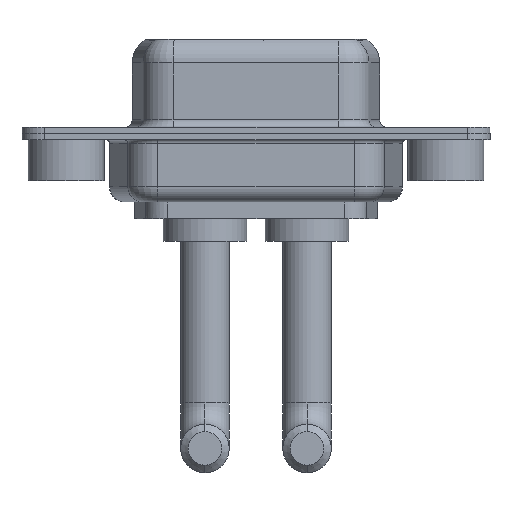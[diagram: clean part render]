
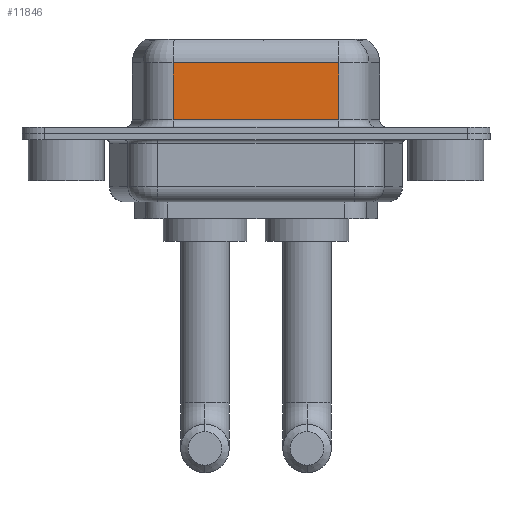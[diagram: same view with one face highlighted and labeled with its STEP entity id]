
A CAD part, front view. The second image highlights one B-rep face of the part: STEP entity #11846.
In plain terms, the highlighted planar face has unit normal (0, -1, 0).
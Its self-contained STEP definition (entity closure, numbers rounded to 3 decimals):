
#338 = CARTESIAN_POINT ( 'NONE',  ( 17.962, -3.95, 0.9 ) ) ;
#714 = VECTOR ( 'NONE', #4623, 1000. ) ;
#788 = VECTOR ( 'NONE', #2277, 1000. ) ;
#857 = CARTESIAN_POINT ( 'NONE',  ( 7.038, -3.95, 6.4 ) ) ;
#1573 = CARTESIAN_POINT ( 'NONE',  ( 17.962, -3.95, 4.65 ) ) ;
#1780 = DIRECTION ( 'NONE',  ( 0., 1., 0. ) ) ;
#1910 = DIRECTION ( 'NONE',  ( -1., 0., 0. ) ) ;
#1981 = EDGE_CURVE ( 'NONE', #7952, #2310, #6005, .T. ) ;
#2015 = ORIENTED_EDGE ( 'NONE', *, *, #2672, .T. ) ;
#2277 = DIRECTION ( 'NONE',  ( 1., 0., 0. ) ) ;
#2310 = VERTEX_POINT ( 'NONE', #12895 ) ;
#2672 = EDGE_CURVE ( 'NONE', #4229, #7952, #9752, .T. ) ;
#2789 = CARTESIAN_POINT ( 'NONE',  ( 17.962, -3.95, 6.4 ) ) ;
#3635 = DIRECTION ( 'NONE',  ( 0., 0., -1. ) ) ;
#3745 = EDGE_CURVE ( 'NONE', #4229, #10550, #6738, .T. ) ;
#3823 = FACE_OUTER_BOUND ( 'NONE', #10102, .T. ) ;
#4229 = VERTEX_POINT ( 'NONE', #10922 ) ;
#4623 = DIRECTION ( 'NONE',  ( -1., 0., 0. ) ) ;
#4859 = ORIENTED_EDGE ( 'NONE', *, *, #11154, .T. ) ;
#4979 = DIRECTION ( 'NONE',  ( 0., 0., -1. ) ) ;
#5725 = CARTESIAN_POINT ( 'NONE',  ( 17.962, -3.95, 6.4 ) ) ;
#6005 = LINE ( 'NONE', #857, #10172 ) ;
#6026 = CARTESIAN_POINT ( 'NONE',  ( 17.962, -3.95, 0.9 ) ) ;
#6738 = LINE ( 'NONE', #5725, #11531 ) ;
#6890 = ORIENTED_EDGE ( 'NONE', *, *, #3745, .F. ) ;
#7952 = VERTEX_POINT ( 'NONE', #9323 ) ;
#9323 = CARTESIAN_POINT ( 'NONE',  ( 7.038, -3.95, 4.65 ) ) ;
#9578 = LINE ( 'NONE', #338, #788 ) ;
#9752 = LINE ( 'NONE', #1573, #714 ) ;
#10002 = ORIENTED_EDGE ( 'NONE', *, *, #1981, .T. ) ;
#10102 = EDGE_LOOP ( 'NONE', ( #6890, #2015, #10002, #4859 ) ) ;
#10172 = VECTOR ( 'NONE', #4979, 1000. ) ;
#10550 = VERTEX_POINT ( 'NONE', #6026 ) ;
#10922 = CARTESIAN_POINT ( 'NONE',  ( 17.962, -3.95, 4.65 ) ) ;
#11154 = EDGE_CURVE ( 'NONE', #2310, #10550, #9578, .T. ) ;
#11531 = VECTOR ( 'NONE', #3635, 1000. ) ;
#11846 = ADVANCED_FACE ( 'NONE', ( #3823 ), #12276, .F. ) ;
#12210 = AXIS2_PLACEMENT_3D ( 'NONE', #2789, #1780, #1910 ) ;
#12276 = PLANE ( 'NONE',  #12210 ) ;
#12895 = CARTESIAN_POINT ( 'NONE',  ( 7.038, -3.95, 0.9 ) ) ;
